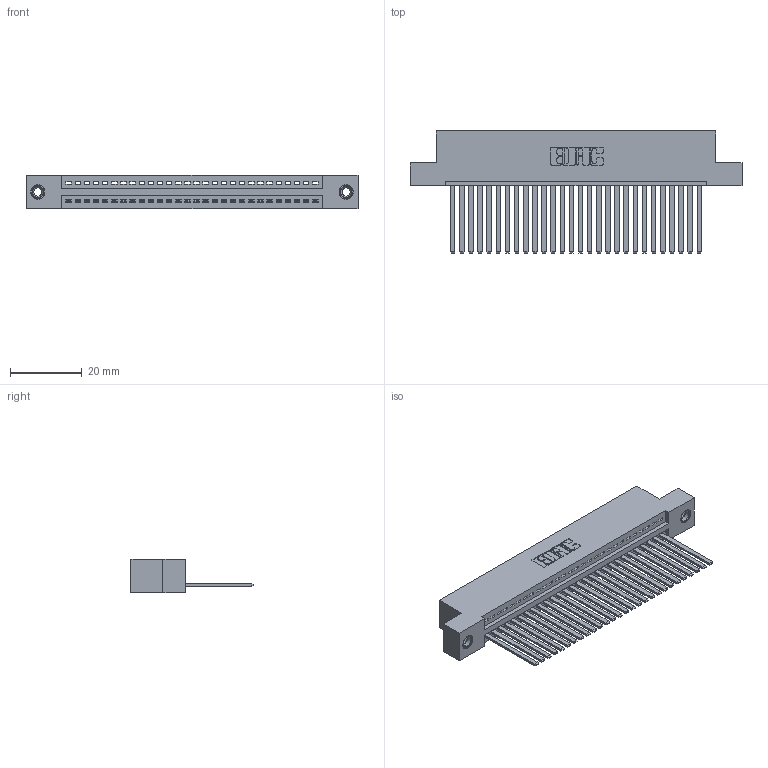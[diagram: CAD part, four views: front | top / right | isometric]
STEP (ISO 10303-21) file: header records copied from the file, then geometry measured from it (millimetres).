
FILE_DESCRIPTION (( 'STEP AP203' ), '1' );
FILE_NAME ('345-028-544-108.STEP', '2019-10-07T06:15:43', ( '' ), ( '' ), 'SwSTEP 2.0', 'SolidWorks 2016', '' );
FILE_SCHEMA (( 'CONFIG_CONTROL_DESIGN' ));
Length unit declared in the file: inch
Products named in the file (4): 345-292-001_345-293-144; 345-028-544-108; 345-250-001_345-250-003-102; 345 Part_Flush Mounting Lugs - 0.156 Dia-TI
Assembly tree (31 placements, depth 2):
  345-028-544-108
    345 Part_Flush Mounting Lugs - 0.156 Dia-TI
    345-292-001_345-293-144  x28
    345-250-001_345-250-003-102  x2
Bounding box: 92.33 x 33.96 x 9.4 mm (x, y, z)
Volume: 8972.6 mm3; surface area: 12726.1 mm2
Topology: 31 solids, 31 shells, 1642 faces, 4901 edges, 3222 vertices
Faces by surface type: plane 1120, cylinder 506, cone 12, torus 4
Entity records: 23960 total; most frequent: CARTESIAN_POINT 4131, ORIENTED_EDGE 4086, DIRECTION 3653, EDGE_CURVE 2043, VECTOR 1783, LINE 1783, VERTEX_POINT 1356, AXIS2_PLACEMENT_3D 935
